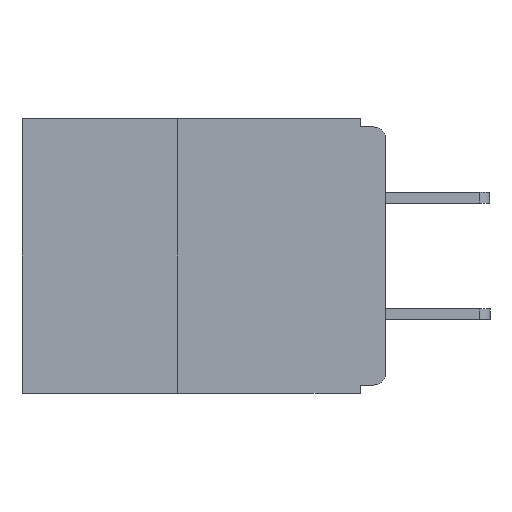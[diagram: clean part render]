
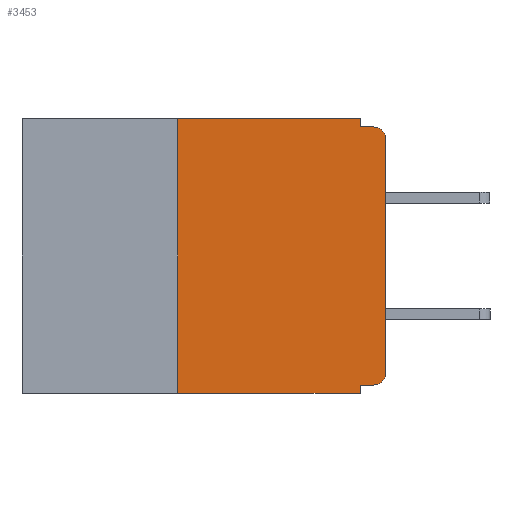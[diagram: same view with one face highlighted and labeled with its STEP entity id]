
A CAD part, left-side view. The second image highlights one B-rep face of the part: STEP entity #3453.
In plain terms, the highlighted planar face has unit normal (-1, 0, 0).
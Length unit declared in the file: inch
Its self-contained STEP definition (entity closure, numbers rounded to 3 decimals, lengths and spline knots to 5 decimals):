
#119 = VERTEX_POINT ( 'NONE', #5995 ) ;
#297 = AXIS2_PLACEMENT_3D ( 'NONE', #1982, #10580, #12378 ) ;
#392 = DIRECTION ( 'NONE',  ( 0., 0., -1. ) ) ;
#400 = VECTOR ( 'NONE', #11461, 39.37008 ) ;
#886 = VERTEX_POINT ( 'NONE', #6045 ) ;
#1118 = FACE_OUTER_BOUND ( 'NONE', #12458, .T. ) ;
#1126 = CIRCLE ( 'NONE', #11727, 0.015 ) ;
#1278 = VECTOR ( 'NONE', #7319, 39.37008 ) ;
#1527 = CARTESIAN_POINT ( 'NONE',  ( 0., 0.015, -0.305 ) ) ;
#1686 = DIRECTION ( 'NONE',  ( -1., 0., 0. ) ) ;
#1701 = DIRECTION ( 'NONE',  ( 0., 0., -1. ) ) ;
#1789 = CARTESIAN_POINT ( 'NONE',  ( 0., 0.437, 0. ) ) ;
#1824 = LINE ( 'NONE', #5973, #7014 ) ;
#1982 = CARTESIAN_POINT ( 'NONE',  ( 0., 0.437, 0. ) ) ;
#2199 = CIRCLE ( 'NONE', #11619, 0.015 ) ;
#2315 = EDGE_CURVE ( 'NONE', #4081, #11848, #1824, .T. ) ;
#2444 = CARTESIAN_POINT ( 'NONE',  ( 0., 0.25, -0.33 ) ) ;
#3008 = EDGE_CURVE ( 'NONE', #4081, #5907, #12384, .T. ) ;
#3453 = ADVANCED_FACE ( 'NONE', ( #1118 ), #6731, .F. ) ;
#3934 = VECTOR ( 'NONE', #11892, 39.37008 ) ;
#4081 = VERTEX_POINT ( 'NONE', #4518 ) ;
#4138 = VERTEX_POINT ( 'NONE', #5361 ) ;
#4258 = DIRECTION ( 'NONE',  ( 0., 0., 1. ) ) ;
#4268 = LINE ( 'NONE', #1789, #3934 ) ;
#4436 = LINE ( 'NONE', #12229, #1278 ) ;
#4473 = VECTOR ( 'NONE', #4258, 39.37008 ) ;
#4477 = EDGE_CURVE ( 'NONE', #13037, #119, #7102, .T. ) ;
#4482 = CARTESIAN_POINT ( 'NONE',  ( 0., 0.015, -0.025 ) ) ;
#4518 = CARTESIAN_POINT ( 'NONE',  ( 0., 0.25, -0.33 ) ) ;
#4895 = LINE ( 'NONE', #8557, #7263 ) ;
#4959 = VERTEX_POINT ( 'NONE', #6467 ) ;
#5253 = ORIENTED_EDGE ( 'NONE', *, *, #11813, .T. ) ;
#5361 = CARTESIAN_POINT ( 'NONE',  ( 0., 0.015, -0.32 ) ) ;
#5477 = DIRECTION ( 'NONE',  ( 0., 0., -1. ) ) ;
#5592 = ORIENTED_EDGE ( 'NONE', *, *, #11226, .T. ) ;
#5804 = ORIENTED_EDGE ( 'NONE', *, *, #10040, .F. ) ;
#5812 = CARTESIAN_POINT ( 'NONE',  ( 0., 0., -0.01 ) ) ;
#5814 = ORIENTED_EDGE ( 'NONE', *, *, #4477, .F. ) ;
#5907 = VERTEX_POINT ( 'NONE', #6260 ) ;
#5913 = ORIENTED_EDGE ( 'NONE', *, *, #12799, .F. ) ;
#5924 = ORIENTED_EDGE ( 'NONE', *, *, #3008, .F. ) ;
#5973 = CARTESIAN_POINT ( 'NONE',  ( 0., 0.437, -0.33 ) ) ;
#5995 = CARTESIAN_POINT ( 'NONE',  ( 0., 0.031, -0.01 ) ) ;
#6040 = ORIENTED_EDGE ( 'NONE', *, *, #2315, .T. ) ;
#6045 = CARTESIAN_POINT ( 'NONE',  ( 0., 0.031, -0.32 ) ) ;
#6050 = VERTEX_POINT ( 'NONE', #12288 ) ;
#6078 = ORIENTED_EDGE ( 'NONE', *, *, #12024, .F. ) ;
#6106 = ORIENTED_EDGE ( 'NONE', *, *, #7052, .F. ) ;
#6169 = ORIENTED_EDGE ( 'NONE', *, *, #6649, .T. ) ;
#6260 = CARTESIAN_POINT ( 'NONE',  ( 0., 0.25, 0. ) ) ;
#6375 = CARTESIAN_POINT ( 'NONE',  ( 0., 0.031, -0.33 ) ) ;
#6467 = CARTESIAN_POINT ( 'NONE',  ( 0., 0., -0.025 ) ) ;
#6649 = EDGE_CURVE ( 'NONE', #4138, #7420, #2199, .T. ) ;
#6731 = PLANE ( 'NONE',  #297 ) ;
#7014 = VECTOR ( 'NONE', #9876, 39.37008 ) ;
#7052 = EDGE_CURVE ( 'NONE', #4138, #886, #8258, .T. ) ;
#7102 = LINE ( 'NONE', #11500, #9964 ) ;
#7263 = VECTOR ( 'NONE', #392, 39.37008 ) ;
#7319 = DIRECTION ( 'NONE',  ( 0., 0., 1. ) ) ;
#7420 = VERTEX_POINT ( 'NONE', #9143 ) ;
#8258 = LINE ( 'NONE', #11530, #400 ) ;
#8557 = CARTESIAN_POINT ( 'NONE',  ( 0., 0.031, -0.33 ) ) ;
#8787 = VECTOR ( 'NONE', #10711, 39.37008 ) ;
#9143 = CARTESIAN_POINT ( 'NONE',  ( 0., 0., -0.305 ) ) ;
#9876 = DIRECTION ( 'NONE',  ( 0., -1., 0. ) ) ;
#9964 = VECTOR ( 'NONE', #10760, 39.37008 ) ;
#10040 = EDGE_CURVE ( 'NONE', #119, #6050, #11767, .T. ) ;
#10580 = DIRECTION ( 'NONE',  ( 1., 0., 0. ) ) ;
#10711 = DIRECTION ( 'NONE',  ( 0., -1., 0. ) ) ;
#10760 = DIRECTION ( 'NONE',  ( 0., 0., -1. ) ) ;
#11226 = EDGE_CURVE ( 'NONE', #4959, #6050, #1126, .T. ) ;
#11402 = DIRECTION ( 'NONE',  ( -1., 0., 0. ) ) ;
#11461 = DIRECTION ( 'NONE',  ( 0., 1., 0. ) ) ;
#11500 = CARTESIAN_POINT ( 'NONE',  ( 0., 0.031, 0. ) ) ;
#11530 = CARTESIAN_POINT ( 'NONE',  ( 0., 0., -0.32 ) ) ;
#11619 = AXIS2_PLACEMENT_3D ( 'NONE', #1527, #1686, #1701 ) ;
#11727 = AXIS2_PLACEMENT_3D ( 'NONE', #4482, #11402, #5477 ) ;
#11767 = LINE ( 'NONE', #5812, #8787 ) ;
#11813 = EDGE_CURVE ( 'NONE', #7420, #4959, #4436, .T. ) ;
#11848 = VERTEX_POINT ( 'NONE', #6375 ) ;
#11892 = DIRECTION ( 'NONE',  ( 0., -1., 0. ) ) ;
#12024 = EDGE_CURVE ( 'NONE', #886, #11848, #4895, .T. ) ;
#12197 = CARTESIAN_POINT ( 'NONE',  ( 0., 0.031, 0. ) ) ;
#12229 = CARTESIAN_POINT ( 'NONE',  ( 0., 0., 0. ) ) ;
#12288 = CARTESIAN_POINT ( 'NONE',  ( 0., 0.015, -0.01 ) ) ;
#12378 = DIRECTION ( 'NONE',  ( 0., 0., -1. ) ) ;
#12384 = LINE ( 'NONE', #2444, #4473 ) ;
#12458 = EDGE_LOOP ( 'NONE', ( #5253, #5592, #5804, #5814, #5913, #5924, #6040, #6078, #6106, #6169 ) ) ;
#12799 = EDGE_CURVE ( 'NONE', #5907, #13037, #4268, .T. ) ;
#13037 = VERTEX_POINT ( 'NONE', #12197 ) ;
